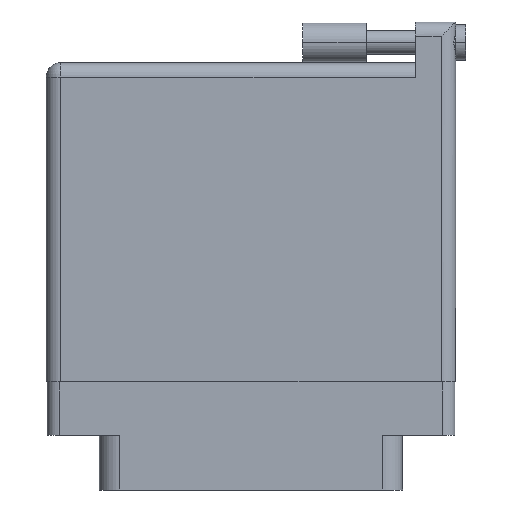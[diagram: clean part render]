
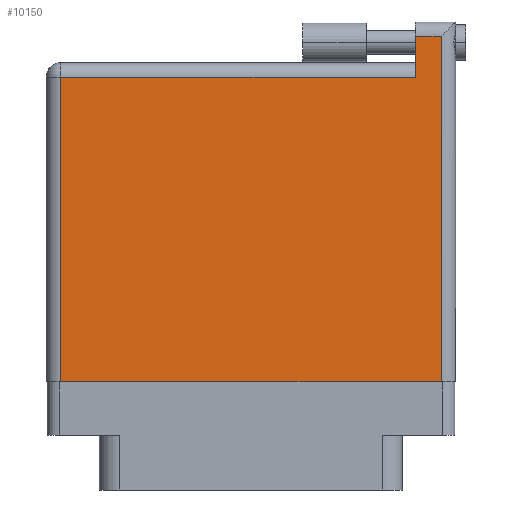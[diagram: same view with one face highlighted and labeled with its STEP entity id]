
A CAD part, front view. The second image highlights one B-rep face of the part: STEP entity #10150.
In plain terms, the highlighted face is planar.
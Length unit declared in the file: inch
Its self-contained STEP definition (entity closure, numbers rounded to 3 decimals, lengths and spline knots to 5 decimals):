
#903 = ORIENTED_EDGE ( 'NONE', *, *, #23433, .T. ) ;
#1050 = EDGE_CURVE ( 'NONE', #34073, #31462, #16844, .T. ) ;
#2608 = VECTOR ( 'NONE', #32443, 39.37008 ) ;
#3255 = CARTESIAN_POINT ( 'NONE',  ( 1.938, 1.766, 0. ) ) ;
#3508 = EDGE_CURVE ( 'NONE', #31462, #14545, #20992, .T. ) ;
#4062 = CARTESIAN_POINT ( 'NONE',  ( 1.811, 1.766, 0. ) ) ;
#5858 = CARTESIAN_POINT ( 'NONE',  ( 0., 1.496, 0. ) ) ;
#6184 = DIRECTION ( 'NONE',  ( -1., 0., 0. ) ) ;
#6405 = DIRECTION ( 'NONE',  ( 0., -1., 0. ) ) ;
#6936 = CARTESIAN_POINT ( 'NONE',  ( 1.811, 1.496, 0. ) ) ;
#8579 = CARTESIAN_POINT ( 'NONE',  ( 1.938, 1.696, 0. ) ) ;
#9402 = DIRECTION ( 'NONE',  ( 0., -1., 0. ) ) ;
#9651 = CARTESIAN_POINT ( 'NONE',  ( 0., 1.566, 0. ) ) ;
#9740 = ORIENTED_EDGE ( 'NONE', *, *, #30497, .T. ) ;
#9753 = CARTESIAN_POINT ( 'NONE',  ( 0., 0., 0. ) ) ;
#9864 = VECTOR ( 'NONE', #6405, 39.37008 ) ;
#10011 = LINE ( 'NONE', #4062, #29200 ) ;
#10150 = ADVANCED_FACE ( 'NONE', ( #19992 ), #25785, .F. ) ;
#10691 = VECTOR ( 'NONE', #15808, 39.37008 ) ;
#10747 = CARTESIAN_POINT ( 'NONE',  ( 1.811, 1.696, 0. ) ) ;
#14294 = VERTEX_POINT ( 'NONE', #6936 ) ;
#14545 = VERTEX_POINT ( 'NONE', #10747 ) ;
#15808 = DIRECTION ( 'NONE',  ( 1., 0., 0. ) ) ;
#16844 = LINE ( 'NONE', #3255, #34410 ) ;
#17631 = ORIENTED_EDGE ( 'NONE', *, *, #1050, .T. ) ;
#17728 = DIRECTION ( 'NONE',  ( -1., 0., 0. ) ) ;
#17818 = LINE ( 'NONE', #9753, #10691 ) ;
#17992 = ORIENTED_EDGE ( 'NONE', *, *, #3508, .T. ) ;
#18652 = CARTESIAN_POINT ( 'NONE',  ( 0., 1.696, 0. ) ) ;
#19412 = EDGE_LOOP ( 'NONE', ( #9740, #17631, #17992, #28481, #903, #29128 ) ) ;
#19992 = FACE_OUTER_BOUND ( 'NONE', #19412, .T. ) ;
#20992 = LINE ( 'NONE', #18652, #28508 ) ;
#21752 = EDGE_CURVE ( 'NONE', #27444, #31467, #28658, .T. ) ;
#23433 = EDGE_CURVE ( 'NONE', #14294, #27444, #34483, .T. ) ;
#23567 = CARTESIAN_POINT ( 'NONE',  ( 1.938, 0., 0. ) ) ;
#24698 = CARTESIAN_POINT ( 'NONE',  ( 0.07, 0., 0. ) ) ;
#24704 = DIRECTION ( 'NONE',  ( 0., 1., 0. ) ) ;
#25785 = PLANE ( 'NONE',  #31507 ) ;
#27444 = VERTEX_POINT ( 'NONE', #28318 ) ;
#28318 = CARTESIAN_POINT ( 'NONE',  ( 0.07, 1.496, 0. ) ) ;
#28481 = ORIENTED_EDGE ( 'NONE', *, *, #34599, .T. ) ;
#28508 = VECTOR ( 'NONE', #6184, 39.37008 ) ;
#28658 = LINE ( 'NONE', #24698, #9864 ) ;
#29128 = ORIENTED_EDGE ( 'NONE', *, *, #21752, .T. ) ;
#29200 = VECTOR ( 'NONE', #9402, 39.37008 ) ;
#29955 = CARTESIAN_POINT ( 'NONE',  ( 0.07, 0., 0. ) ) ;
#30497 = EDGE_CURVE ( 'NONE', #31467, #34073, #17818, .T. ) ;
#31013 = DIRECTION ( 'NONE',  ( 0., 0., -1. ) ) ;
#31462 = VERTEX_POINT ( 'NONE', #8579 ) ;
#31467 = VERTEX_POINT ( 'NONE', #29955 ) ;
#31507 = AXIS2_PLACEMENT_3D ( 'NONE', #9651, #31013, #17728 ) ;
#32443 = DIRECTION ( 'NONE',  ( -1., 0., 0. ) ) ;
#34073 = VERTEX_POINT ( 'NONE', #23567 ) ;
#34410 = VECTOR ( 'NONE', #24704, 39.37008 ) ;
#34483 = LINE ( 'NONE', #5858, #2608 ) ;
#34599 = EDGE_CURVE ( 'NONE', #14545, #14294, #10011, .T. ) ;
